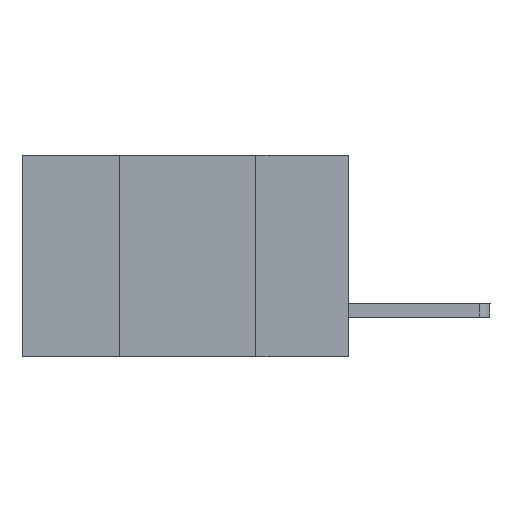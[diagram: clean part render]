
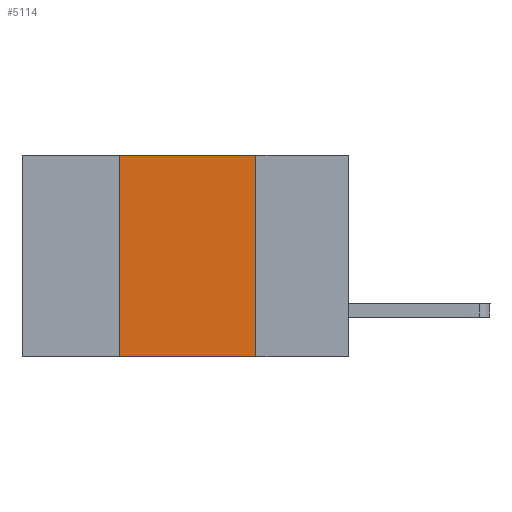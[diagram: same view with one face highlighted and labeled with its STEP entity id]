
A CAD part, left-side view. The second image highlights one B-rep face of the part: STEP entity #5114.
In plain terms, the highlighted planar face has unit normal (-1, 0, 0).
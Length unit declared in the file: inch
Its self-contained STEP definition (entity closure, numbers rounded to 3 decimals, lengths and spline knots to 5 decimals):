
#462 = CARTESIAN_POINT ( 'NONE',  ( 0., 0.42, 0. ) ) ;
#1733 = CARTESIAN_POINT ( 'NONE',  ( 0., 0.6, 0. ) ) ;
#1737 = EDGE_CURVE ( 'NONE', #5082, #4347, #1977, .T. ) ;
#1857 = ORIENTED_EDGE ( 'NONE', *, *, #3747, .T. ) ;
#1977 = LINE ( 'NONE', #8257, #5087 ) ;
#2158 = ORIENTED_EDGE ( 'NONE', *, *, #8133, .F. ) ;
#2420 = ORIENTED_EDGE ( 'NONE', *, *, #1737, .F. ) ;
#2475 = LINE ( 'NONE', #8600, #3840 ) ;
#3022 = CARTESIAN_POINT ( 'NONE',  ( 0., 0.42, -0.37 ) ) ;
#3115 = DIRECTION ( 'NONE',  ( 0., -1., 0. ) ) ;
#3454 = VECTOR ( 'NONE', #5963, 39.37008 ) ;
#3528 = CARTESIAN_POINT ( 'NONE',  ( 0., 0.17, 0. ) ) ;
#3747 = EDGE_CURVE ( 'NONE', #5082, #4555, #2475, .T. ) ;
#3840 = VECTOR ( 'NONE', #7867, 39.37008 ) ;
#3920 = FACE_OUTER_BOUND ( 'NONE', #4244, .T. ) ;
#3960 = PLANE ( 'NONE',  #6902 ) ;
#4244 = EDGE_LOOP ( 'NONE', ( #2158, #7822, #2420, #1857 ) ) ;
#4347 = VERTEX_POINT ( 'NONE', #462 ) ;
#4506 = DIRECTION ( 'NONE',  ( 0., 0., -1. ) ) ;
#4555 = VERTEX_POINT ( 'NONE', #6352 ) ;
#4707 = DIRECTION ( 'NONE',  ( 0., 0., 1. ) ) ;
#5082 = VERTEX_POINT ( 'NONE', #3022 ) ;
#5087 = VECTOR ( 'NONE', #4707, 39.37008 ) ;
#5114 = ADVANCED_FACE ( 'NONE', ( #3920 ), #3960, .F. ) ;
#5147 = EDGE_CURVE ( 'NONE', #4347, #7897, #5371, .T. ) ;
#5341 = VECTOR ( 'NONE', #3115, 39.37008 ) ;
#5371 = LINE ( 'NONE', #1733, #5341 ) ;
#5963 = DIRECTION ( 'NONE',  ( 0., 0., -1. ) ) ;
#6352 = CARTESIAN_POINT ( 'NONE',  ( 0., 0.17, -0.37 ) ) ;
#6705 = DIRECTION ( 'NONE',  ( 1., 0., 0. ) ) ;
#6808 = LINE ( 'NONE', #7333, #3454 ) ;
#6902 = AXIS2_PLACEMENT_3D ( 'NONE', #7926, #6705, #4506 ) ;
#7333 = CARTESIAN_POINT ( 'NONE',  ( 0., 0.17, -0.37 ) ) ;
#7822 = ORIENTED_EDGE ( 'NONE', *, *, #5147, .F. ) ;
#7867 = DIRECTION ( 'NONE',  ( 0., -1., 0. ) ) ;
#7897 = VERTEX_POINT ( 'NONE', #3528 ) ;
#7926 = CARTESIAN_POINT ( 'NONE',  ( 0., 0.6, 0. ) ) ;
#8133 = EDGE_CURVE ( 'NONE', #7897, #4555, #6808, .T. ) ;
#8257 = CARTESIAN_POINT ( 'NONE',  ( 0., 0.42, -0.37 ) ) ;
#8600 = CARTESIAN_POINT ( 'NONE',  ( 0., 0.6, -0.37 ) ) ;
